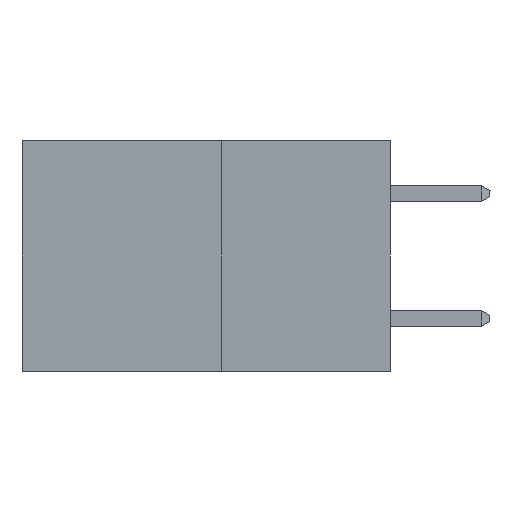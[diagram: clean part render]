
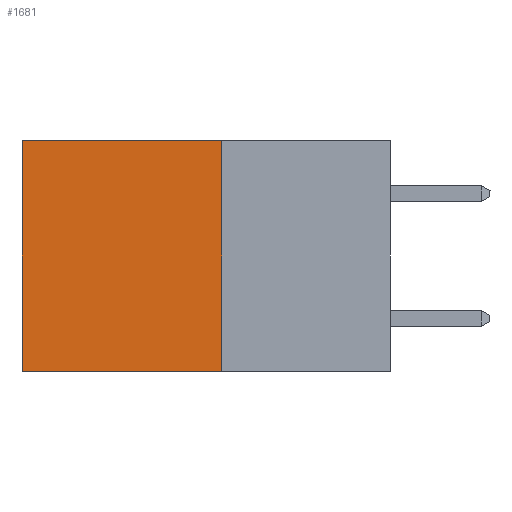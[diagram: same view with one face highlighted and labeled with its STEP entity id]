
A CAD part, left-side view. The second image highlights one B-rep face of the part: STEP entity #1681.
In plain terms, the highlighted planar face has unit normal (-1, 0, 0).
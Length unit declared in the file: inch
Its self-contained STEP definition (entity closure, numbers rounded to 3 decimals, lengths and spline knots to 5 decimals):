
#44 = CARTESIAN_POINT ( 'NONE',  ( 0.277, 0.27, 0. ) ) ;
#300 = EDGE_CURVE ( 'NONE', #5069, #2846, #1036, .T. ) ;
#399 = DIRECTION ( 'NONE',  ( 0., 0., -1. ) ) ;
#558 = VERTEX_POINT ( 'NONE', #5491 ) ;
#1036 = LINE ( 'NONE', #2339, #5161 ) ;
#1108 = CARTESIAN_POINT ( 'NONE',  ( 0.277, 0.59, 0. ) ) ;
#1117 = EDGE_CURVE ( 'NONE', #558, #2722, #8978, .T. ) ;
#1429 = CARTESIAN_POINT ( 'NONE',  ( 0.277, 0.59, -0.37 ) ) ;
#1673 = DIRECTION ( 'NONE',  ( 1., 0., 0. ) ) ;
#1681 = ADVANCED_FACE ( 'NONE', ( #7618 ), #5838, .F. ) ;
#2339 = CARTESIAN_POINT ( 'NONE',  ( 0.277, 0.27, 0. ) ) ;
#2586 = EDGE_CURVE ( 'NONE', #2846, #2722, #6014, .T. ) ;
#2722 = VERTEX_POINT ( 'NONE', #1429 ) ;
#2846 = VERTEX_POINT ( 'NONE', #1108 ) ;
#3216 = ORIENTED_EDGE ( 'NONE', *, *, #8999, .F. ) ;
#3457 = CARTESIAN_POINT ( 'NONE',  ( 0.277, 0.27, -0.37 ) ) ;
#3551 = CARTESIAN_POINT ( 'NONE',  ( 0.277, 0.59, -0.37 ) ) ;
#3683 = DIRECTION ( 'NONE',  ( 0., 1., 0. ) ) ;
#3810 = DIRECTION ( 'NONE',  ( 0., 0., -1. ) ) ;
#3906 = DIRECTION ( 'NONE',  ( 0., 0., -1. ) ) ;
#3952 = VECTOR ( 'NONE', #3906, 39.37008 ) ;
#4333 = ORIENTED_EDGE ( 'NONE', *, *, #1117, .F. ) ;
#4561 = VECTOR ( 'NONE', #399, 39.37008 ) ;
#4890 = AXIS2_PLACEMENT_3D ( 'NONE', #3457, #1673, #3810 ) ;
#5069 = VERTEX_POINT ( 'NONE', #44 ) ;
#5161 = VECTOR ( 'NONE', #3683, 39.37008 ) ;
#5491 = CARTESIAN_POINT ( 'NONE',  ( 0.277, 0.27, -0.37 ) ) ;
#5640 = EDGE_LOOP ( 'NONE', ( #9277, #4333, #3216, #8707 ) ) ;
#5838 = PLANE ( 'NONE',  #4890 ) ;
#6014 = LINE ( 'NONE', #3551, #3952 ) ;
#6829 = VECTOR ( 'NONE', #6955, 39.37008 ) ;
#6900 = CARTESIAN_POINT ( 'NONE',  ( 0.277, 0.27, -0.37 ) ) ;
#6955 = DIRECTION ( 'NONE',  ( 0., 1., 0. ) ) ;
#7618 = FACE_OUTER_BOUND ( 'NONE', #5640, .T. ) ;
#8213 = LINE ( 'NONE', #6900, #4561 ) ;
#8707 = ORIENTED_EDGE ( 'NONE', *, *, #300, .T. ) ;
#8978 = LINE ( 'NONE', #9241, #6829 ) ;
#8999 = EDGE_CURVE ( 'NONE', #5069, #558, #8213, .T. ) ;
#9241 = CARTESIAN_POINT ( 'NONE',  ( 0.277, 0.27, -0.37 ) ) ;
#9277 = ORIENTED_EDGE ( 'NONE', *, *, #2586, .T. ) ;
